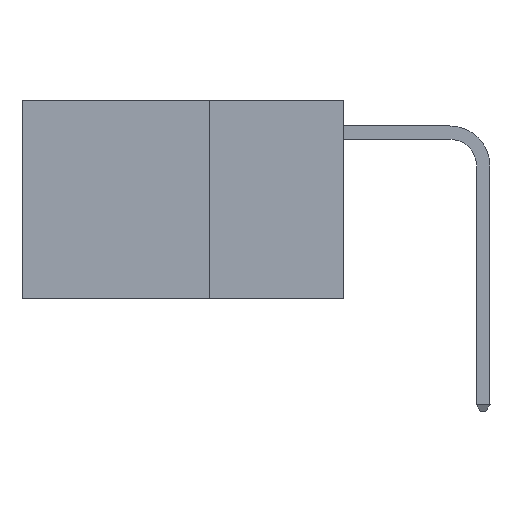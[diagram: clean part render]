
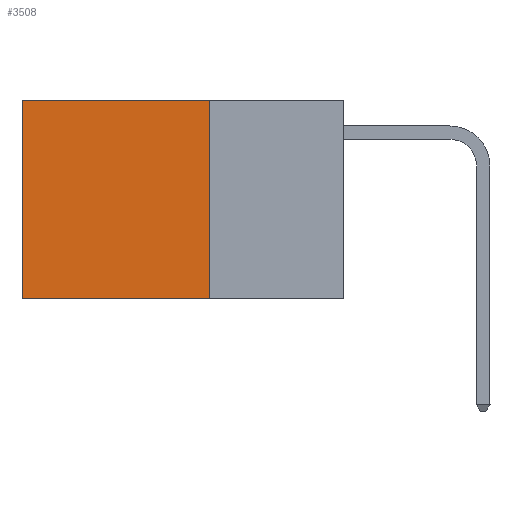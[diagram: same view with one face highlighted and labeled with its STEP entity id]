
A CAD part, left-side view. The second image highlights one B-rep face of the part: STEP entity #3508.
In plain terms, the highlighted planar face has unit normal (-1, 0, 0).
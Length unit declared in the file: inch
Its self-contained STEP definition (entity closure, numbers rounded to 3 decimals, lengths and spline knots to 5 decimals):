
#479 = CARTESIAN_POINT ( 'NONE',  ( 0.2625, 0.6, 0. ) ) ;
#506 = CARTESIAN_POINT ( 'NONE',  ( 0.2625, 0.25, 0. ) ) ;
#846 = ORIENTED_EDGE ( 'NONE', *, *, #12058, .F. ) ;
#1063 = VERTEX_POINT ( 'NONE', #12056 ) ;
#2244 = PLANE ( 'NONE',  #3068 ) ;
#2426 = ORIENTED_EDGE ( 'NONE', *, *, #8392, .T. ) ;
#2856 = CARTESIAN_POINT ( 'NONE',  ( 0.2625, 0.25, -0.37 ) ) ;
#3068 = AXIS2_PLACEMENT_3D ( 'NONE', #14648, #8823, #12601 ) ;
#3178 = CARTESIAN_POINT ( 'NONE',  ( 0.2625, 0.25, 0. ) ) ;
#3226 = FACE_OUTER_BOUND ( 'NONE', #12041, .T. ) ;
#3508 = ADVANCED_FACE ( 'NONE', ( #3226 ), #2244, .F. ) ;
#4044 = ORIENTED_EDGE ( 'NONE', *, *, #7058, .T. ) ;
#4572 = VERTEX_POINT ( 'NONE', #13294 ) ;
#4646 = VERTEX_POINT ( 'NONE', #2856 ) ;
#4732 = LINE ( 'NONE', #506, #14570 ) ;
#5629 = DIRECTION ( 'NONE',  ( 0., 1., 0. ) ) ;
#5919 = LINE ( 'NONE', #11695, #12857 ) ;
#6173 = LINE ( 'NONE', #479, #7323 ) ;
#6663 = EDGE_CURVE ( 'NONE', #12988, #4646, #4732, .T. ) ;
#6966 = DIRECTION ( 'NONE',  ( 0., 1., 0. ) ) ;
#7058 = EDGE_CURVE ( 'NONE', #1063, #4572, #6173, .T. ) ;
#7323 = VECTOR ( 'NONE', #14105, 39.37008 ) ;
#8392 = EDGE_CURVE ( 'NONE', #12988, #1063, #8775, .T. ) ;
#8775 = LINE ( 'NONE', #3178, #9506 ) ;
#8823 = DIRECTION ( 'NONE',  ( 1., 0., 0. ) ) ;
#9252 = DIRECTION ( 'NONE',  ( 0., 0., -1. ) ) ;
#9506 = VECTOR ( 'NONE', #5629, 39.37008 ) ;
#11331 = CARTESIAN_POINT ( 'NONE',  ( 0.2625, 0.25, 0. ) ) ;
#11462 = ORIENTED_EDGE ( 'NONE', *, *, #6663, .F. ) ;
#11695 = CARTESIAN_POINT ( 'NONE',  ( 0.2625, 0.25, -0.37 ) ) ;
#12041 = EDGE_LOOP ( 'NONE', ( #4044, #846, #11462, #2426 ) ) ;
#12056 = CARTESIAN_POINT ( 'NONE',  ( 0.2625, 0.6, 0. ) ) ;
#12058 = EDGE_CURVE ( 'NONE', #4646, #4572, #5919, .T. ) ;
#12601 = DIRECTION ( 'NONE',  ( 0., 0., -1. ) ) ;
#12857 = VECTOR ( 'NONE', #6966, 39.37008 ) ;
#12988 = VERTEX_POINT ( 'NONE', #11331 ) ;
#13294 = CARTESIAN_POINT ( 'NONE',  ( 0.2625, 0.6, -0.37 ) ) ;
#14105 = DIRECTION ( 'NONE',  ( 0., 0., -1. ) ) ;
#14570 = VECTOR ( 'NONE', #9252, 39.37008 ) ;
#14648 = CARTESIAN_POINT ( 'NONE',  ( 0.2625, 0.25, 0. ) ) ;
